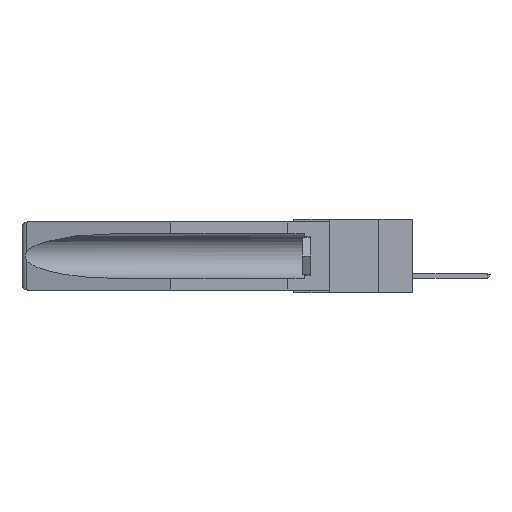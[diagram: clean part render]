
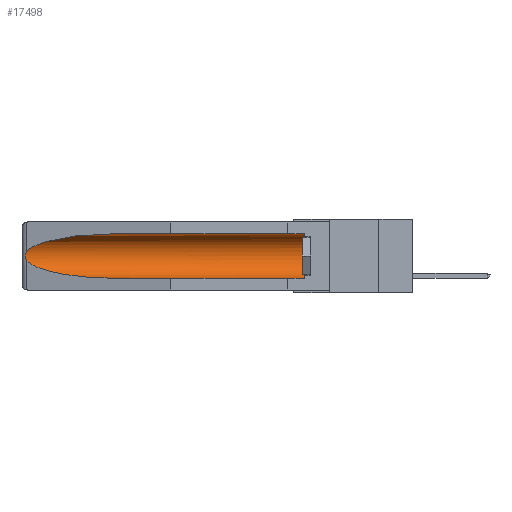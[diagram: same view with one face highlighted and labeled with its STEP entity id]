
A CAD part, left-side view. The second image highlights one B-rep face of the part: STEP entity #17498.
In plain terms, the highlighted cylindrical face has radius 2.857 mm (diameter 5.715 mm), a partial arc.
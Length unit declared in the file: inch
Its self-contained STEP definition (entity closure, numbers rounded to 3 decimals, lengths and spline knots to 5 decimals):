
#429 = VECTOR ( 'NONE', #23582, 39.37008 ) ;
#1023 = ORIENTED_EDGE ( 'NONE', *, *, #21910, .T. ) ;
#1633 = CARTESIAN_POINT ( 'NONE',  ( 0.2675, 1.53308, -0.17534 ) ) ;
#1812 = CARTESIAN_POINT ( 'NONE',  ( 0.26537, 1.52718, -0.14972 ) ) ;
#1914 = CARTESIAN_POINT ( 'NONE',  ( 0.26597, 1.52961, -0.15275 ) ) ;
#2231 = LINE ( 'NONE', #6595, #9972 ) ;
#3135 = CARTESIAN_POINT ( 'NONE',  ( 0.155, -0.30754, -0.1715 ) ) ;
#3596 = CARTESIAN_POINT ( 'NONE',  ( 0.2673, 1.53269, -0.17917 ) ) ;
#3812 = CARTESIAN_POINT ( 'NONE',  ( 0.26537, 1.52718, -0.14972 ) ) ;
#3872 = CARTESIAN_POINT ( 'NONE',  ( 0.2673, 1.5327, -0.16383 ) ) ;
#4793 = CARTESIAN_POINT ( 'NONE',  ( 0.155, 1.07973, -0.059 ) ) ;
#4822 = CARTESIAN_POINT ( 'NONE',  ( 0.155, 1.07973, -0.284 ) ) ;
#4836 = VERTEX_POINT ( 'NONE', #3812 ) ;
#5033 = EDGE_LOOP ( 'NONE', ( #13060, #1023, #16073, #15947, #15881, #18911 ) ) ;
#5764 = CARTESIAN_POINT ( 'NONE',  ( 0.26655, 1.53094, -0.18657 ) ) ;
#6212 =( BOUNDED_CURVE ( )  B_SPLINE_CURVE ( 3, ( #7977, #13993, #26120, #4822 ),
 .UNSPECIFIED., .F., .F. ) 
 B_SPLINE_CURVE_WITH_KNOTS ( ( 4, 4 ),
 ( 0.1948, 1.5708 ),
 .UNSPECIFIED. ) 
 CURVE ( )  GEOMETRIC_REPRESENTATION_ITEM ( )  RATIONAL_B_SPLINE_CURVE ( ( 1., 0.848, 0.848, 1. ) ) 
 REPRESENTATION_ITEM ( '' )  );
#6595 = CARTESIAN_POINT ( 'NONE',  ( 0.155, -0.30754, -0.284 ) ) ;
#6975 = CARTESIAN_POINT ( 'NONE',  ( 0.21114, 1.30732, -0.059 ) ) ;
#7482 = CIRCLE ( 'NONE', #12564, 0.1125 ) ;
#7747 = VERTEX_POINT ( 'NONE', #16005 ) ;
#7950 = CARTESIAN_POINT ( 'NONE',  ( 0.26654, 1.53092, -0.15636 ) ) ;
#7977 = CARTESIAN_POINT ( 'NONE',  ( 0.26537, 1.52718, -0.19328 ) ) ;
#8730 = CARTESIAN_POINT ( 'NONE',  ( 0.155, -0.30754, -0.059 ) ) ;
#8850 = CARTESIAN_POINT ( 'NONE',  ( 0.25451, 1.48313, -0.09465 ) ) ;
#9419 = CYLINDRICAL_SURFACE ( 'NONE', #12832, 0.1125 ) ;
#9972 = VECTOR ( 'NONE', #21663, 39.37008 ) ;
#10079 = CARTESIAN_POINT ( 'NONE',  ( 0.26597, 1.5296, -0.19026 ) ) ;
#11602 = CARTESIAN_POINT ( 'NONE',  ( 0.155, 0.126, -0.284 ) ) ;
#11626 = DIRECTION ( 'NONE',  ( 0., 1., 0. ) ) ;
#11908 = VERTEX_POINT ( 'NONE', #18533 ) ;
#12467 = FACE_OUTER_BOUND ( 'NONE', #5033, .T. ) ;
#12564 = AXIS2_PLACEMENT_3D ( 'NONE', #22686, #13954, #26666 ) ;
#12832 = AXIS2_PLACEMENT_3D ( 'NONE', #3135, #11626, #14043 ) ;
#13060 = ORIENTED_EDGE ( 'NONE', *, *, #17861, .T. ) ;
#13358 = EDGE_CURVE ( 'NONE', #7747, #22516, #26877, .T. ) ;
#13469 = CARTESIAN_POINT ( 'NONE',  ( 0.26537, 1.52718, -0.14972 ) ) ;
#13954 = DIRECTION ( 'NONE',  ( 0., -1., 0. ) ) ;
#13993 = CARTESIAN_POINT ( 'NONE',  ( 0.25451, 1.48313, -0.24835 ) ) ;
#14043 = DIRECTION ( 'NONE',  ( 0., 0., 1. ) ) ;
#15881 = ORIENTED_EDGE ( 'NONE', *, *, #23831, .T. ) ;
#15947 = ORIENTED_EDGE ( 'NONE', *, *, #21760, .F. ) ;
#16005 = CARTESIAN_POINT ( 'NONE',  ( 0.155, 0.126, -0.059 ) ) ;
#16073 = ORIENTED_EDGE ( 'NONE', *, *, #24172, .T. ) ;
#16503 = VERTEX_POINT ( 'NONE', #11602 ) ;
#17498 = ADVANCED_FACE ( 'NONE', ( #12467 ), #9419, .F. ) ;
#17861 = EDGE_CURVE ( 'NONE', #22516, #4836, #19110, .T. ) ;
#18533 = CARTESIAN_POINT ( 'NONE',  ( 0.26537, 1.52718, -0.19328 ) ) ;
#18559 = CARTESIAN_POINT ( 'NONE',  ( 0.155, 1.07973, -0.059 ) ) ;
#18812 = CARTESIAN_POINT ( 'NONE',  ( 0.2675, 1.53308, -0.16763 ) ) ;
#18911 = ORIENTED_EDGE ( 'NONE', *, *, #13358, .T. ) ;
#19110 =( BOUNDED_CURVE ( )  B_SPLINE_CURVE ( 3, ( #4793, #6975, #8850, #13469 ),
 .UNSPECIFIED., .F., .F. ) 
 B_SPLINE_CURVE_WITH_KNOTS ( ( 4, 4 ),
 ( 4.71239, 6.08839 ),
 .UNSPECIFIED. ) 
 CURVE ( )  GEOMETRIC_REPRESENTATION_ITEM ( )  RATIONAL_B_SPLINE_CURVE ( ( 1., 0.848, 0.848, 1. ) ) 
 REPRESENTATION_ITEM ( '' )  );
#19839 = CARTESIAN_POINT ( 'NONE',  ( 0.155, 1.07973, -0.284 ) ) ;
#21663 = DIRECTION ( 'NONE',  ( 0., 1., 0. ) ) ;
#21760 = EDGE_CURVE ( 'NONE', #16503, #26174, #2231, .T. ) ;
#21910 = EDGE_CURVE ( 'NONE', #4836, #11908, #21988, .T. ) ;
#21988 = B_SPLINE_CURVE_WITH_KNOTS ( 'NONE', 3,
 ( #1812, #1914, #7950, #3872, #18812, #1633, #3596, #5764, #10079, #25000 ),
 .UNSPECIFIED., .F., .F.,
 ( 4, 2, 2, 2, 4 ),
 ( 0., 0.00029, 0.00058, 0.00087, 0.00117 ),
 .UNSPECIFIED. ) ;
#22516 = VERTEX_POINT ( 'NONE', #18559 ) ;
#22686 = CARTESIAN_POINT ( 'NONE',  ( 0.155, 0.126, -0.1715 ) ) ;
#23582 = DIRECTION ( 'NONE',  ( 0., 1., 0. ) ) ;
#23831 = EDGE_CURVE ( 'NONE', #16503, #7747, #7482, .T. ) ;
#24172 = EDGE_CURVE ( 'NONE', #11908, #26174, #6212, .T. ) ;
#25000 = CARTESIAN_POINT ( 'NONE',  ( 0.26537, 1.52718, -0.19328 ) ) ;
#26120 = CARTESIAN_POINT ( 'NONE',  ( 0.21114, 1.30732, -0.284 ) ) ;
#26174 = VERTEX_POINT ( 'NONE', #19839 ) ;
#26666 = DIRECTION ( 'NONE',  ( 0., 0., 1. ) ) ;
#26877 = LINE ( 'NONE', #8730, #429 ) ;
